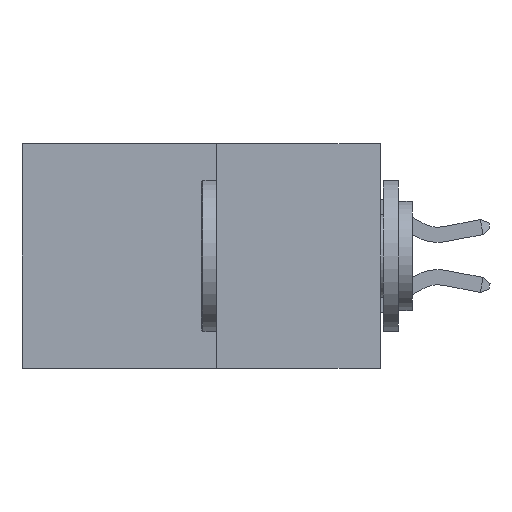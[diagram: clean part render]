
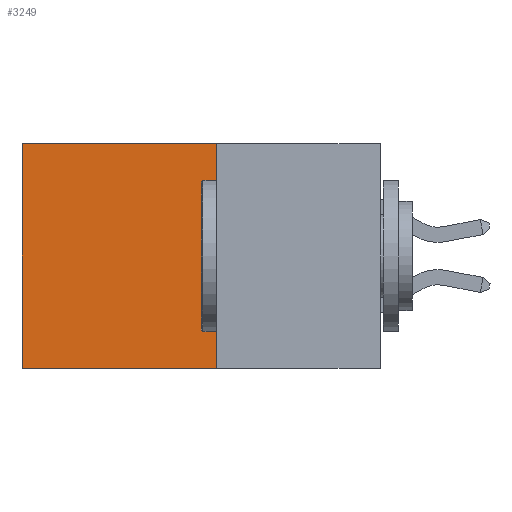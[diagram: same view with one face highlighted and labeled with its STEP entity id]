
A CAD part, left-side view. The second image highlights one B-rep face of the part: STEP entity #3249.
In plain terms, the highlighted planar face has unit normal (-1, 0, 0).
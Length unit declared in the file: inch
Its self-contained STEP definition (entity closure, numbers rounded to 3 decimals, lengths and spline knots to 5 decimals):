
#453 = PLANE ( 'NONE',  #3305 ) ;
#1568 = EDGE_CURVE ( 'NONE', #19565, #6213, #19825, .T. ) ;
#3173 = VECTOR ( 'NONE', #10594, 39.37008 ) ;
#3249 = ADVANCED_FACE ( 'NONE', ( #9633 ), #453, .F. ) ;
#3305 = AXIS2_PLACEMENT_3D ( 'NONE', #19396, #20484, #20413 ) ;
#3542 = EDGE_CURVE ( 'NONE', #6213, #18295, #7370, .T. ) ;
#4381 = DIRECTION ( 'NONE',  ( 0., 0., -1. ) ) ;
#5546 = EDGE_CURVE ( 'NONE', #19565, #12484, #13573, .T. ) ;
#6213 = VERTEX_POINT ( 'NONE', #11472 ) ;
#6696 = LINE ( 'NONE', #15546, #15210 ) ;
#7211 = VECTOR ( 'NONE', #13044, 39.37008 ) ;
#7370 = LINE ( 'NONE', #10986, #3173 ) ;
#9316 = VECTOR ( 'NONE', #18924, 39.37008 ) ;
#9605 = ORIENTED_EDGE ( 'NONE', *, *, #12531, .T. ) ;
#9633 = FACE_OUTER_BOUND ( 'NONE', #18762, .T. ) ;
#10594 = DIRECTION ( 'NONE',  ( 0., 1., 0. ) ) ;
#10633 = CARTESIAN_POINT ( 'NONE',  ( 0.277, 0.59, 0. ) ) ;
#10660 = CARTESIAN_POINT ( 'NONE',  ( 0.277, 0.27, -0.37 ) ) ;
#10986 = CARTESIAN_POINT ( 'NONE',  ( 0.277, 0.27, -0.37 ) ) ;
#11472 = CARTESIAN_POINT ( 'NONE',  ( 0.277, 0.27, -0.37 ) ) ;
#12461 = ORIENTED_EDGE ( 'NONE', *, *, #3542, .F. ) ;
#12484 = VERTEX_POINT ( 'NONE', #10633 ) ;
#12531 = EDGE_CURVE ( 'NONE', #12484, #18295, #6696, .T. ) ;
#13044 = DIRECTION ( 'NONE',  ( 0., 0., -1. ) ) ;
#13573 = LINE ( 'NONE', #18967, #9316 ) ;
#14258 = ORIENTED_EDGE ( 'NONE', *, *, #1568, .F. ) ;
#15210 = VECTOR ( 'NONE', #4381, 39.37008 ) ;
#15546 = CARTESIAN_POINT ( 'NONE',  ( 0.277, 0.59, -0.37 ) ) ;
#16650 = ORIENTED_EDGE ( 'NONE', *, *, #5546, .T. ) ;
#18053 = CARTESIAN_POINT ( 'NONE',  ( 0.277, 0.27, 0. ) ) ;
#18295 = VERTEX_POINT ( 'NONE', #18625 ) ;
#18625 = CARTESIAN_POINT ( 'NONE',  ( 0.277, 0.59, -0.37 ) ) ;
#18762 = EDGE_LOOP ( 'NONE', ( #9605, #12461, #14258, #16650 ) ) ;
#18924 = DIRECTION ( 'NONE',  ( 0., 1., 0. ) ) ;
#18967 = CARTESIAN_POINT ( 'NONE',  ( 0.277, 0.27, 0. ) ) ;
#19396 = CARTESIAN_POINT ( 'NONE',  ( 0.277, 0.27, -0.37 ) ) ;
#19565 = VERTEX_POINT ( 'NONE', #18053 ) ;
#19825 = LINE ( 'NONE', #10660, #7211 ) ;
#20413 = DIRECTION ( 'NONE',  ( 0., 0., -1. ) ) ;
#20484 = DIRECTION ( 'NONE',  ( 1., 0., 0. ) ) ;
